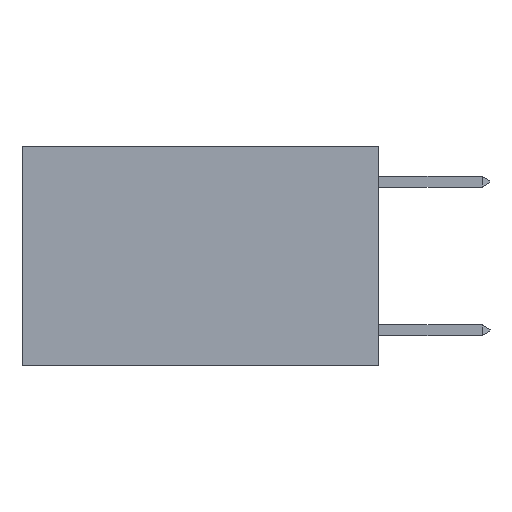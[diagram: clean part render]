
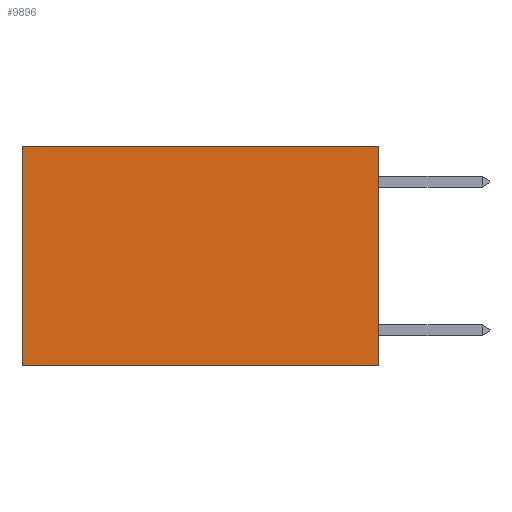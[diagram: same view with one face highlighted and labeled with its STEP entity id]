
A CAD part, left-side view. The second image highlights one B-rep face of the part: STEP entity #9896.
In plain terms, the highlighted planar face has unit normal (-1, 0, 0).
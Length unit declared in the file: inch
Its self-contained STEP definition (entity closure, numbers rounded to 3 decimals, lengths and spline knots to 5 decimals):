
#754 = CARTESIAN_POINT ( 'NONE',  ( 0.2625, 0., -0.37 ) ) ;
#983 = EDGE_CURVE ( 'NONE', #14425, #11556, #17168, .T. ) ;
#1145 = FACE_OUTER_BOUND ( 'NONE', #12770, .T. ) ;
#2591 = EDGE_CURVE ( 'NONE', #11556, #7236, #9532, .T. ) ;
#4085 = DIRECTION ( 'NONE',  ( 0., 0., -1. ) ) ;
#4870 = ORIENTED_EDGE ( 'NONE', *, *, #16508, .T. ) ;
#4897 = AXIS2_PLACEMENT_3D ( 'NONE', #16160, #15278, #15272 ) ;
#5915 = LINE ( 'NONE', #16086, #9129 ) ;
#7165 = DIRECTION ( 'NONE',  ( 0., 1., 0. ) ) ;
#7236 = VERTEX_POINT ( 'NONE', #16555 ) ;
#7614 = VERTEX_POINT ( 'NONE', #19486 ) ;
#8378 = CARTESIAN_POINT ( 'NONE',  ( 0.2625, 0., 0. ) ) ;
#8510 = ORIENTED_EDGE ( 'NONE', *, *, #983, .F. ) ;
#9129 = VECTOR ( 'NONE', #7165, 39.37008 ) ;
#9532 = LINE ( 'NONE', #10140, #9625 ) ;
#9625 = VECTOR ( 'NONE', #9791, 39.37008 ) ;
#9791 = DIRECTION ( 'NONE',  ( 0., 1., 0. ) ) ;
#9896 = ADVANCED_FACE ( 'NONE', ( #1145 ), #15574, .F. ) ;
#10140 = CARTESIAN_POINT ( 'NONE',  ( 0.2625, 0., -0.37 ) ) ;
#10254 = VECTOR ( 'NONE', #4085, 39.37008 ) ;
#11030 = LINE ( 'NONE', #14639, #10254 ) ;
#11556 = VERTEX_POINT ( 'NONE', #754 ) ;
#12770 = EDGE_LOOP ( 'NONE', ( #4870, #13773, #8510, #14648 ) ) ;
#13386 = CARTESIAN_POINT ( 'NONE',  ( 0.2625, 0., 0. ) ) ;
#13773 = ORIENTED_EDGE ( 'NONE', *, *, #2591, .F. ) ;
#14425 = VERTEX_POINT ( 'NONE', #8378 ) ;
#14639 = CARTESIAN_POINT ( 'NONE',  ( 0.2625, 0.6, 0. ) ) ;
#14648 = ORIENTED_EDGE ( 'NONE', *, *, #15861, .T. ) ;
#15272 = DIRECTION ( 'NONE',  ( 0., 0., -1. ) ) ;
#15278 = DIRECTION ( 'NONE',  ( 1., 0., 0. ) ) ;
#15574 = PLANE ( 'NONE',  #4897 ) ;
#15861 = EDGE_CURVE ( 'NONE', #14425, #7614, #5915, .T. ) ;
#16086 = CARTESIAN_POINT ( 'NONE',  ( 0.2625, 0., 0. ) ) ;
#16160 = CARTESIAN_POINT ( 'NONE',  ( 0.2625, 0., 0. ) ) ;
#16508 = EDGE_CURVE ( 'NONE', #7614, #7236, #11030, .T. ) ;
#16555 = CARTESIAN_POINT ( 'NONE',  ( 0.2625, 0.6, -0.37 ) ) ;
#16697 = DIRECTION ( 'NONE',  ( 0., 0., -1. ) ) ;
#17011 = VECTOR ( 'NONE', #16697, 39.37008 ) ;
#17168 = LINE ( 'NONE', #13386, #17011 ) ;
#19486 = CARTESIAN_POINT ( 'NONE',  ( 0.2625, 0.6, 0. ) ) ;
